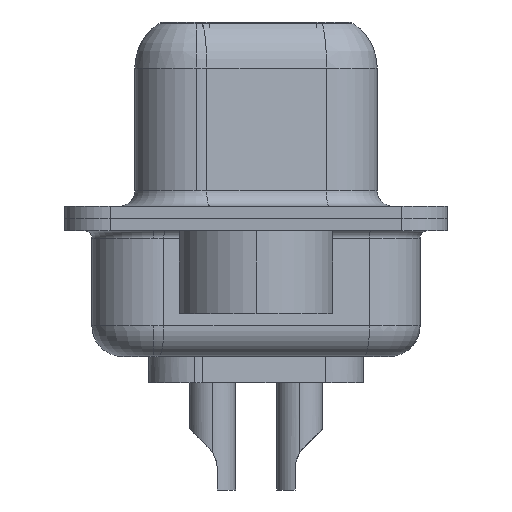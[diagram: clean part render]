
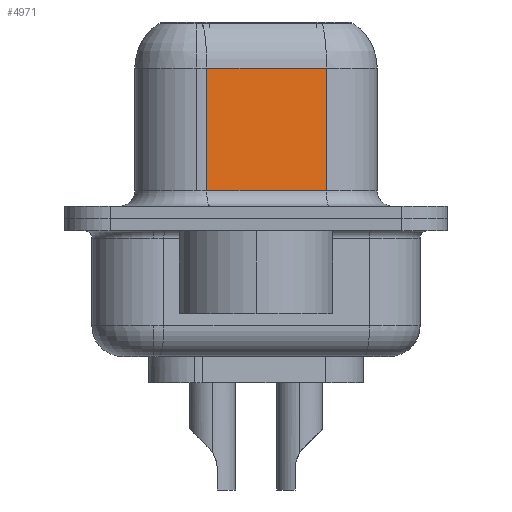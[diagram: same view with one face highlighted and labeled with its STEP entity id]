
A CAD part, left-side view. The second image highlights one B-rep face of the part: STEP entity #4971.
In plain terms, the highlighted planar face has unit normal (-0.985, -0.174, 0).
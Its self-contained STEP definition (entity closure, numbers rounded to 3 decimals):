
#538 = PLANE ( 'NONE',  #7038 ) ;
#652 = CARTESIAN_POINT ( 'NONE',  ( 5.043, -2.297, 6.65 ) ) ;
#1026 = VERTEX_POINT ( 'NONE', #6119 ) ;
#1473 = VERTEX_POINT ( 'NONE', #4897 ) ;
#1655 = ORIENTED_EDGE ( 'NONE', *, *, #18608, .T. ) ;
#2675 = VECTOR ( 'NONE', #17468, 1000. ) ;
#2899 = VECTOR ( 'NONE', #10191, 1000. ) ;
#4128 = ORIENTED_EDGE ( 'NONE', *, *, #10645, .T. ) ;
#4897 = CARTESIAN_POINT ( 'NONE',  ( 4.355, 1.603, 0.9 ) ) ;
#4971 = ADVANCED_FACE ( 'NONE', ( #15247 ), #538, .F. ) ;
#5064 = VECTOR ( 'NONE', #7487, 1000. ) ;
#5654 = DIRECTION ( 'NONE',  ( -0.174, 0.985, 0. ) ) ;
#6119 = CARTESIAN_POINT ( 'NONE',  ( 5.043, -2.297, 4.9 ) ) ;
#7038 = AXIS2_PLACEMENT_3D ( 'NONE', #652, #21002, #5654 ) ;
#7199 = EDGE_CURVE ( 'NONE', #8794, #1473, #15958, .T. ) ;
#7487 = DIRECTION ( 'NONE',  ( 0., 0., -1. ) ) ;
#8074 = DIRECTION ( 'NONE',  ( 0.174, -0.985, 0. ) ) ;
#8170 = CARTESIAN_POINT ( 'NONE',  ( 5.043, -2.297, 0.9 ) ) ;
#8794 = VERTEX_POINT ( 'NONE', #11832 ) ;
#9009 = LINE ( 'NONE', #19348, #2675 ) ;
#9077 = VECTOR ( 'NONE', #8074, 1000. ) ;
#10191 = DIRECTION ( 'NONE',  ( 0., 0., -1. ) ) ;
#10645 = EDGE_CURVE ( 'NONE', #1026, #8794, #9009, .T. ) ;
#11832 = CARTESIAN_POINT ( 'NONE',  ( 4.355, 1.603, 4.9 ) ) ;
#12458 = ORIENTED_EDGE ( 'NONE', *, *, #7199, .T. ) ;
#13306 = EDGE_LOOP ( 'NONE', ( #15287, #4128, #12458, #1655 ) ) ;
#13414 = CARTESIAN_POINT ( 'NONE',  ( 5.043, -2.297, 0.9 ) ) ;
#14209 = EDGE_CURVE ( 'NONE', #1026, #20692, #15208, .T. ) ;
#14403 = CARTESIAN_POINT ( 'NONE',  ( 4.355, 1.603, 6.65 ) ) ;
#15079 = LINE ( 'NONE', #13414, #9077 ) ;
#15208 = LINE ( 'NONE', #18858, #2899 ) ;
#15247 = FACE_OUTER_BOUND ( 'NONE', #13306, .T. ) ;
#15287 = ORIENTED_EDGE ( 'NONE', *, *, #14209, .F. ) ;
#15958 = LINE ( 'NONE', #14403, #5064 ) ;
#17468 = DIRECTION ( 'NONE',  ( -0.174, 0.985, 0. ) ) ;
#18608 = EDGE_CURVE ( 'NONE', #1473, #20692, #15079, .T. ) ;
#18858 = CARTESIAN_POINT ( 'NONE',  ( 5.043, -2.297, 6.65 ) ) ;
#19348 = CARTESIAN_POINT ( 'NONE',  ( 5.043, -2.297, 4.9 ) ) ;
#20692 = VERTEX_POINT ( 'NONE', #8170 ) ;
#21002 = DIRECTION ( 'NONE',  ( 0.985, 0.174, 0. ) ) ;
